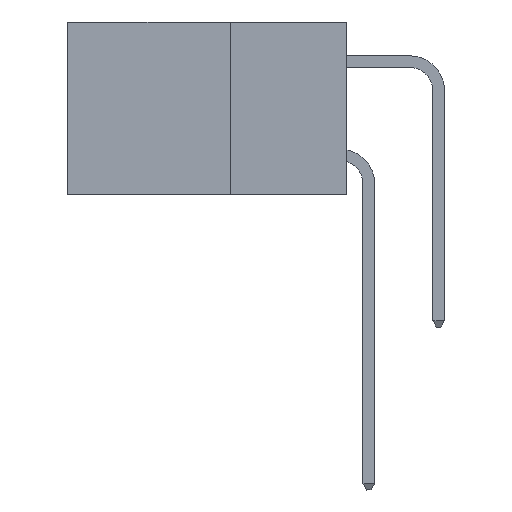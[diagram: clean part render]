
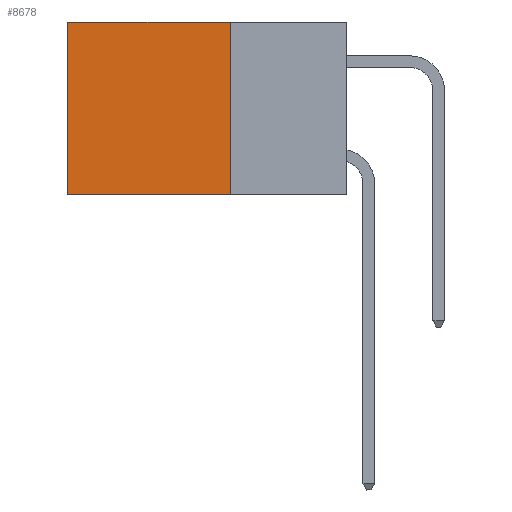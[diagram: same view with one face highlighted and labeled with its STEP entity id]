
A CAD part, left-side view. The second image highlights one B-rep face of the part: STEP entity #8678.
In plain terms, the highlighted planar face has unit normal (-1, 0, 0).
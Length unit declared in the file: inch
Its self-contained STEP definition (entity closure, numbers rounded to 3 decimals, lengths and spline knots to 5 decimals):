
#1642 = ORIENTED_EDGE ( 'NONE', *, *, #28368, .T. ) ;
#2910 = AXIS2_PLACEMENT_3D ( 'NONE', #14862, #6469, #32379 ) ;
#3224 = PLANE ( 'NONE',  #2910 ) ;
#3718 = VECTOR ( 'NONE', #22486, 39.37008 ) ;
#3971 = CARTESIAN_POINT ( 'NONE',  ( 0.2875, 0.25, -0.37 ) ) ;
#6469 = DIRECTION ( 'NONE',  ( 1., 0., 0. ) ) ;
#7471 = CARTESIAN_POINT ( 'NONE',  ( 0.2875, 0.25, 0. ) ) ;
#8678 = ADVANCED_FACE ( 'NONE', ( #36132 ), #3224, .F. ) ;
#10672 = EDGE_CURVE ( 'NONE', #12725, #20272, #22599, .T. ) ;
#10811 = DIRECTION ( 'NONE',  ( 0., 1., 0. ) ) ;
#10813 = VECTOR ( 'NONE', #32436, 39.37008 ) ;
#11023 = VECTOR ( 'NONE', #23535, 39.37008 ) ;
#11899 = LINE ( 'NONE', #17630, #11023 ) ;
#12671 = ORIENTED_EDGE ( 'NONE', *, *, #31088, .T. ) ;
#12725 = VERTEX_POINT ( 'NONE', #7471 ) ;
#14862 = CARTESIAN_POINT ( 'NONE',  ( 0.2875, 0.25, 0. ) ) ;
#16528 = LINE ( 'NONE', #25859, #16965 ) ;
#16676 = CARTESIAN_POINT ( 'NONE',  ( 0.2875, 0.6, 0. ) ) ;
#16965 = VECTOR ( 'NONE', #10811, 39.37008 ) ;
#17630 = CARTESIAN_POINT ( 'NONE',  ( 0.2875, 0.25, -0.37 ) ) ;
#19074 = CARTESIAN_POINT ( 'NONE',  ( 0.2875, 0.6, 0. ) ) ;
#19989 = EDGE_LOOP ( 'NONE', ( #12671, #36944, #29410, #1642 ) ) ;
#20272 = VERTEX_POINT ( 'NONE', #3971 ) ;
#22486 = DIRECTION ( 'NONE',  ( 0., 0., -1. ) ) ;
#22599 = LINE ( 'NONE', #37069, #10813 ) ;
#23535 = DIRECTION ( 'NONE',  ( 0., 1., 0. ) ) ;
#25859 = CARTESIAN_POINT ( 'NONE',  ( 0.2875, 0.25, 0. ) ) ;
#26690 = VERTEX_POINT ( 'NONE', #33494 ) ;
#27398 = EDGE_CURVE ( 'NONE', #20272, #26690, #11899, .T. ) ;
#28368 = EDGE_CURVE ( 'NONE', #12725, #31570, #16528, .T. ) ;
#29410 = ORIENTED_EDGE ( 'NONE', *, *, #10672, .F. ) ;
#31088 = EDGE_CURVE ( 'NONE', #31570, #26690, #33531, .T. ) ;
#31570 = VERTEX_POINT ( 'NONE', #16676 ) ;
#32379 = DIRECTION ( 'NONE',  ( 0., 0., -1. ) ) ;
#32436 = DIRECTION ( 'NONE',  ( 0., 0., -1. ) ) ;
#33494 = CARTESIAN_POINT ( 'NONE',  ( 0.2875, 0.6, -0.37 ) ) ;
#33531 = LINE ( 'NONE', #19074, #3718 ) ;
#36132 = FACE_OUTER_BOUND ( 'NONE', #19989, .T. ) ;
#36944 = ORIENTED_EDGE ( 'NONE', *, *, #27398, .F. ) ;
#37069 = CARTESIAN_POINT ( 'NONE',  ( 0.2875, 0.25, 0. ) ) ;
